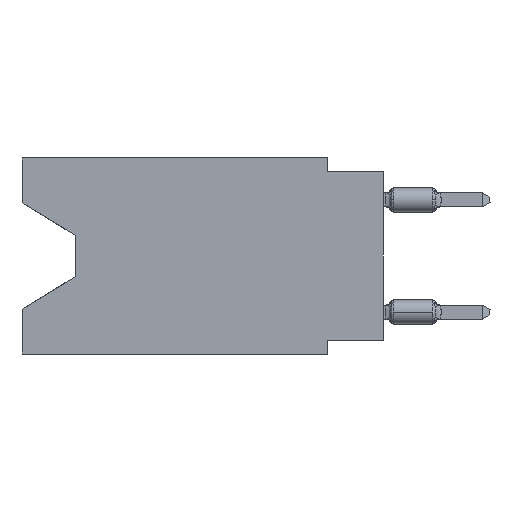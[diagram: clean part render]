
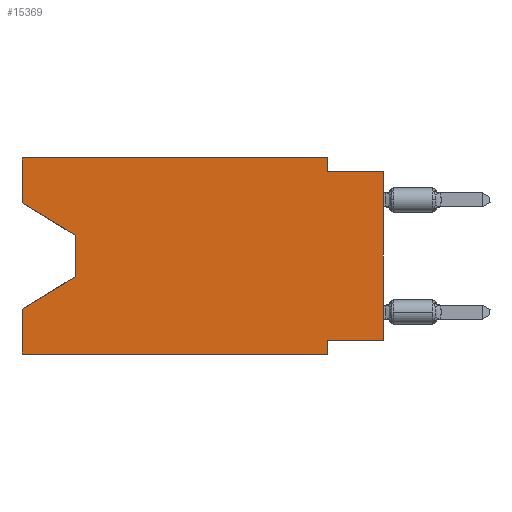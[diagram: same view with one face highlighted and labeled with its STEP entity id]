
A CAD part, left-side view. The second image highlights one B-rep face of the part: STEP entity #15369.
In plain terms, the highlighted planar face has unit normal (-1, 0, 0).
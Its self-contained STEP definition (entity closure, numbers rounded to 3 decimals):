
#947 = VERTEX_POINT ( 'NONE', #17429 ) ;
#1042 = VERTEX_POINT ( 'NONE', #8139 ) ;
#1467 = CARTESIAN_POINT ( 'NONE',  ( 0., 16.383, -2.038 ) ) ;
#1699 = CARTESIAN_POINT ( 'NONE',  ( 0., 2.54, -8.255 ) ) ;
#2519 = DIRECTION ( 'NONE',  ( 0., -1., 0. ) ) ;
#2598 = DIRECTION ( 'NONE',  ( 0., 1., 0. ) ) ;
#2821 = VECTOR ( 'NONE', #14932, 1000. ) ;
#4096 = CARTESIAN_POINT ( 'NONE',  ( 0., 0., 0. ) ) ;
#4617 = LINE ( 'NONE', #31724, #2821 ) ;
#5544 = CARTESIAN_POINT ( 'NONE',  ( 0., 16.383, -8.89 ) ) ;
#5815 = EDGE_LOOP ( 'NONE', ( #7907, #8762, #47118, #9502, #66563, #10172, #15002, #22206, #23315, #62893, #39487, #54748 ) ) ;
#6722 = DIRECTION ( 'NONE',  ( 0., 0., 1. ) ) ;
#7290 = VERTEX_POINT ( 'NONE', #9313 ) ;
#7907 = ORIENTED_EDGE ( 'NONE', *, *, #64919, .T. ) ;
#8139 = CARTESIAN_POINT ( 'NONE',  ( 0., 16.383, -2.038 ) ) ;
#8451 = VECTOR ( 'NONE', #2519, 1000. ) ;
#8552 = EDGE_CURVE ( 'NONE', #7290, #61858, #39076, .T. ) ;
#8648 = DIRECTION ( 'NONE',  ( 0., 0., -1. ) ) ;
#8762 = ORIENTED_EDGE ( 'NONE', *, *, #10025, .T. ) ;
#9313 = CARTESIAN_POINT ( 'NONE',  ( 0., 2.54, -0.635 ) ) ;
#9502 = ORIENTED_EDGE ( 'NONE', *, *, #27213, .F. ) ;
#10025 = EDGE_CURVE ( 'NONE', #35517, #54304, #49670, .T. ) ;
#10172 = ORIENTED_EDGE ( 'NONE', *, *, #15419, .F. ) ;
#10807 = VERTEX_POINT ( 'NONE', #5544 ) ;
#10989 = DIRECTION ( 'NONE',  ( 0., 0., 1. ) ) ;
#11475 = DIRECTION ( 'NONE',  ( 0., 0., -1. ) ) ;
#11885 = EDGE_CURVE ( 'NONE', #15934, #61858, #42611, .T. ) ;
#12588 = CARTESIAN_POINT ( 'NONE',  ( 0., 16.383, 0. ) ) ;
#13211 = CARTESIAN_POINT ( 'NONE',  ( 0., 16.383, -8.89 ) ) ;
#13902 = VECTOR ( 'NONE', #47856, 1000. ) ;
#14010 = VECTOR ( 'NONE', #69370, 1000. ) ;
#14397 = LINE ( 'NONE', #68276, #42617 ) ;
#14932 = DIRECTION ( 'NONE',  ( 0., 0., -1. ) ) ;
#15002 = ORIENTED_EDGE ( 'NONE', *, *, #15378, .F. ) ;
#15369 = ADVANCED_FACE ( 'NONE', ( #44020 ), #55785, .F. ) ;
#15378 = EDGE_CURVE ( 'NONE', #15934, #45605, #41461, .T. ) ;
#15419 = EDGE_CURVE ( 'NONE', #45605, #947, #46099, .T. ) ;
#15934 = VERTEX_POINT ( 'NONE', #68413 ) ;
#17429 = CARTESIAN_POINT ( 'NONE',  ( 0., 2.54, -8.89 ) ) ;
#21843 = CARTESIAN_POINT ( 'NONE',  ( 0., 13.97, -3.505 ) ) ;
#22206 = ORIENTED_EDGE ( 'NONE', *, *, #11885, .T. ) ;
#22729 = VERTEX_POINT ( 'NONE', #52925 ) ;
#23315 = ORIENTED_EDGE ( 'NONE', *, *, #8552, .F. ) ;
#23567 = LINE ( 'NONE', #1467, #31542 ) ;
#23647 = CARTESIAN_POINT ( 'NONE',  ( 0., 16.383, 0. ) ) ;
#24008 = CARTESIAN_POINT ( 'NONE',  ( 0., 2.54, -8.89 ) ) ;
#24448 = LINE ( 'NONE', #61936, #55693 ) ;
#25409 = CARTESIAN_POINT ( 'NONE',  ( 0., 13.97, -3.505 ) ) ;
#27213 = EDGE_CURVE ( 'NONE', #10807, #22729, #38108, .T. ) ;
#28079 = VECTOR ( 'NONE', #2598, 1000. ) ;
#31542 = VECTOR ( 'NONE', #62113, 1000. ) ;
#31724 = CARTESIAN_POINT ( 'NONE',  ( 0., 2.54, 0. ) ) ;
#33434 = VECTOR ( 'NONE', #11475, 1000. ) ;
#34375 = DIRECTION ( 'NONE',  ( 1., 0., 0. ) ) ;
#35517 = VERTEX_POINT ( 'NONE', #25409 ) ;
#37098 = EDGE_CURVE ( 'NONE', #63828, #59337, #24448, .T. ) ;
#38108 = LINE ( 'NONE', #59899, #40864 ) ;
#39076 = LINE ( 'NONE', #55495, #13902 ) ;
#39487 = ORIENTED_EDGE ( 'NONE', *, *, #37098, .F. ) ;
#39939 = CARTESIAN_POINT ( 'NONE',  ( 0., 13.97, -5.385 ) ) ;
#40501 = DIRECTION ( 'NONE',  ( 0., -1., 0. ) ) ;
#40573 = AXIS2_PLACEMENT_3D ( 'NONE', #12588, #34375, #51136 ) ;
#40864 = VECTOR ( 'NONE', #10989, 1000. ) ;
#41461 = LINE ( 'NONE', #63223, #28079 ) ;
#42611 = LINE ( 'NONE', #4096, #14010 ) ;
#42617 = VECTOR ( 'NONE', #57948, 1000. ) ;
#43975 = EDGE_CURVE ( 'NONE', #1042, #63828, #55600, .T. ) ;
#44020 = FACE_OUTER_BOUND ( 'NONE', #5815, .T. ) ;
#45605 = VERTEX_POINT ( 'NONE', #1699 ) ;
#46099 = LINE ( 'NONE', #24008, #57768 ) ;
#47118 = ORIENTED_EDGE ( 'NONE', *, *, #47404, .T. ) ;
#47404 = EDGE_CURVE ( 'NONE', #54304, #22729, #14397, .T. ) ;
#47856 = DIRECTION ( 'NONE',  ( 0., -1., 0. ) ) ;
#49201 = CARTESIAN_POINT ( 'NONE',  ( 0., 16.383, 0. ) ) ;
#49670 = LINE ( 'NONE', #21843, #33434 ) ;
#50852 = CARTESIAN_POINT ( 'NONE',  ( 0., 0., -0.635 ) ) ;
#51136 = DIRECTION ( 'NONE',  ( 0., 0., -1. ) ) ;
#52925 = CARTESIAN_POINT ( 'NONE',  ( 0., 16.383, -6.852 ) ) ;
#54304 = VERTEX_POINT ( 'NONE', #39939 ) ;
#54748 = ORIENTED_EDGE ( 'NONE', *, *, #43975, .F. ) ;
#55495 = CARTESIAN_POINT ( 'NONE',  ( 0., 0., -0.635 ) ) ;
#55600 = LINE ( 'NONE', #49201, #65282 ) ;
#55693 = VECTOR ( 'NONE', #40501, 1000. ) ;
#55785 = PLANE ( 'NONE',  #40573 ) ;
#56038 = LINE ( 'NONE', #13211, #8451 ) ;
#56954 = CARTESIAN_POINT ( 'NONE',  ( 0., 2.54, 0. ) ) ;
#57133 = EDGE_CURVE ( 'NONE', #59337, #7290, #4617, .T. ) ;
#57768 = VECTOR ( 'NONE', #8648, 1000. ) ;
#57948 = DIRECTION ( 'NONE',  ( 0., 0.855, -0.519 ) ) ;
#59337 = VERTEX_POINT ( 'NONE', #56954 ) ;
#59899 = CARTESIAN_POINT ( 'NONE',  ( 0., 16.383, 0. ) ) ;
#61858 = VERTEX_POINT ( 'NONE', #50852 ) ;
#61936 = CARTESIAN_POINT ( 'NONE',  ( 0., 16.383, 0. ) ) ;
#62113 = DIRECTION ( 'NONE',  ( 0., -0.855, -0.519 ) ) ;
#62893 = ORIENTED_EDGE ( 'NONE', *, *, #57133, .F. ) ;
#63223 = CARTESIAN_POINT ( 'NONE',  ( 0., 0., -8.255 ) ) ;
#63828 = VERTEX_POINT ( 'NONE', #23647 ) ;
#64919 = EDGE_CURVE ( 'NONE', #1042, #35517, #23567, .T. ) ;
#65282 = VECTOR ( 'NONE', #6722, 1000. ) ;
#66563 = ORIENTED_EDGE ( 'NONE', *, *, #68245, .T. ) ;
#68245 = EDGE_CURVE ( 'NONE', #10807, #947, #56038, .T. ) ;
#68276 = CARTESIAN_POINT ( 'NONE',  ( 0., 13.97, -5.385 ) ) ;
#68413 = CARTESIAN_POINT ( 'NONE',  ( 0., 0., -8.255 ) ) ;
#69370 = DIRECTION ( 'NONE',  ( 0., 0., 1. ) ) ;
